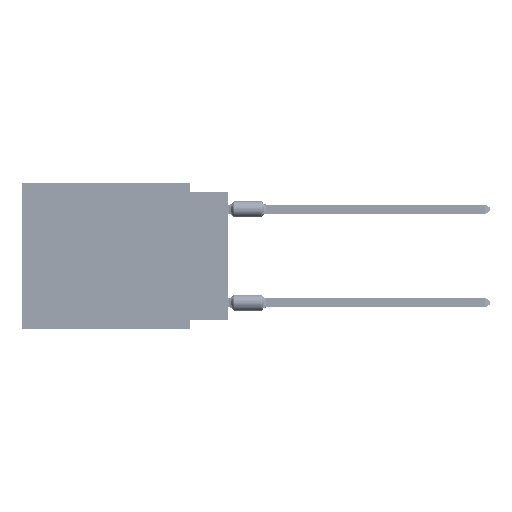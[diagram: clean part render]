
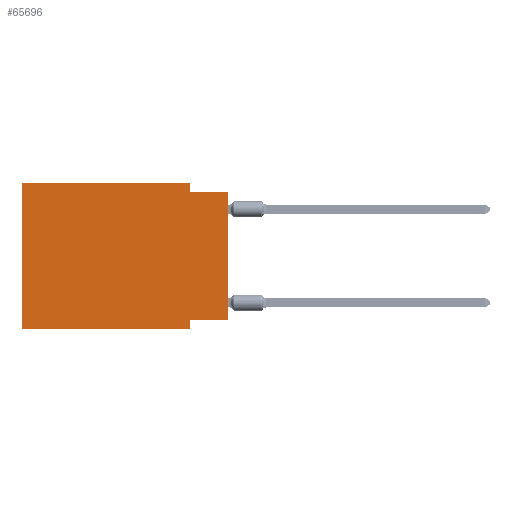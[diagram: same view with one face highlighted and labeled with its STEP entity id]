
A CAD part, left-side view. The second image highlights one B-rep face of the part: STEP entity #65696.
In plain terms, the highlighted planar face has unit normal (-1, 0, 0).
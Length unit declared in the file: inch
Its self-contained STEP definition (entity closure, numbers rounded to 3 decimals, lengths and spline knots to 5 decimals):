
#1277 = VECTOR ( 'NONE', #46324, 39.37008 ) ;
#2667 = EDGE_CURVE ( 'NONE', #44023, #79629, #66763, .T. ) ;
#2785 = VERTEX_POINT ( 'NONE', #69150 ) ;
#5005 = CARTESIAN_POINT ( 'NONE',  ( 0., 0.1, -0.39 ) ) ;
#6451 = CARTESIAN_POINT ( 'NONE',  ( 0., 0., -0.025 ) ) ;
#6894 = DIRECTION ( 'NONE',  ( 0., 0., -1. ) ) ;
#7888 = FACE_OUTER_BOUND ( 'NONE', #57667, .T. ) ;
#8982 = VECTOR ( 'NONE', #80253, 39.37008 ) ;
#9087 = CARTESIAN_POINT ( 'NONE',  ( 0., 0.55, -0.39 ) ) ;
#9197 = VERTEX_POINT ( 'NONE', #6451 ) ;
#11913 = CARTESIAN_POINT ( 'NONE',  ( 0., 0.1, -0.39 ) ) ;
#16998 = ORIENTED_EDGE ( 'NONE', *, *, #53743, .T. ) ;
#19771 = EDGE_CURVE ( 'NONE', #75054, #43557, #27640, .T. ) ;
#20317 = DIRECTION ( 'NONE',  ( 0., -1., 0. ) ) ;
#20482 = CARTESIAN_POINT ( 'NONE',  ( 0., 0.55, 0. ) ) ;
#20891 = ORIENTED_EDGE ( 'NONE', *, *, #31232, .T. ) ;
#21186 = CARTESIAN_POINT ( 'NONE',  ( 0., 0.55, -0.39 ) ) ;
#21458 = VERTEX_POINT ( 'NONE', #79711 ) ;
#21685 = VERTEX_POINT ( 'NONE', #21186 ) ;
#22049 = CARTESIAN_POINT ( 'NONE',  ( 0., 0.55, 0. ) ) ;
#22130 = CARTESIAN_POINT ( 'NONE',  ( 0., 0.1, -0.365 ) ) ;
#23485 = ORIENTED_EDGE ( 'NONE', *, *, #50300, .F. ) ;
#24976 = DIRECTION ( 'NONE',  ( 0., 0., -1. ) ) ;
#25943 = ORIENTED_EDGE ( 'NONE', *, *, #36119, .F. ) ;
#27640 = LINE ( 'NONE', #52410, #1277 ) ;
#31041 = LINE ( 'NONE', #42805, #70798 ) ;
#31232 = EDGE_CURVE ( 'NONE', #21458, #9197, #31041, .T. ) ;
#31469 = DIRECTION ( 'NONE',  ( 1., 0., 0. ) ) ;
#32112 = LINE ( 'NONE', #75944, #61336 ) ;
#32636 = VECTOR ( 'NONE', #52434, 39.37008 ) ;
#35011 = VECTOR ( 'NONE', #35903, 39.37008 ) ;
#35903 = DIRECTION ( 'NONE',  ( 0., 0., -1. ) ) ;
#36119 = EDGE_CURVE ( 'NONE', #21685, #75054, #77206, .T. ) ;
#37667 = EDGE_CURVE ( 'NONE', #2785, #9197, #32112, .T. ) ;
#38570 = LINE ( 'NONE', #68635, #79699 ) ;
#41069 = ORIENTED_EDGE ( 'NONE', *, *, #2667, .F. ) ;
#41079 = ORIENTED_EDGE ( 'NONE', *, *, #19771, .F. ) ;
#42036 = ORIENTED_EDGE ( 'NONE', *, *, #73039, .F. ) ;
#42805 = CARTESIAN_POINT ( 'NONE',  ( 0., 0., 0. ) ) ;
#43557 = VERTEX_POINT ( 'NONE', #51895 ) ;
#44023 = VERTEX_POINT ( 'NONE', #22130 ) ;
#45892 = LINE ( 'NONE', #61178, #8982 ) ;
#46324 = DIRECTION ( 'NONE',  ( 0., -1., 0. ) ) ;
#50300 = EDGE_CURVE ( 'NONE', #43557, #2785, #38570, .T. ) ;
#50542 = PLANE ( 'NONE',  #79718 ) ;
#51895 = CARTESIAN_POINT ( 'NONE',  ( 0., 0.1, 0. ) ) ;
#52410 = CARTESIAN_POINT ( 'NONE',  ( 0., 0.55, 0. ) ) ;
#52434 = DIRECTION ( 'NONE',  ( 0., 0., 1. ) ) ;
#53743 = EDGE_CURVE ( 'NONE', #21685, #79629, #58218, .T. ) ;
#55807 = DIRECTION ( 'NONE',  ( 0., 0., 1. ) ) ;
#57667 = EDGE_LOOP ( 'NONE', ( #20891, #70760, #23485, #41079, #25943, #16998, #41069, #42036 ) ) ;
#58218 = LINE ( 'NONE', #9087, #65632 ) ;
#61178 = CARTESIAN_POINT ( 'NONE',  ( 0., 0., -0.365 ) ) ;
#61336 = VECTOR ( 'NONE', #20317, 39.37008 ) ;
#65632 = VECTOR ( 'NONE', #70412, 39.37008 ) ;
#65696 = ADVANCED_FACE ( 'NONE', ( #7888 ), #50542, .F. ) ;
#66240 = CARTESIAN_POINT ( 'NONE',  ( 0., 0.55, 0. ) ) ;
#66763 = LINE ( 'NONE', #11913, #35011 ) ;
#68635 = CARTESIAN_POINT ( 'NONE',  ( 0., 0.1, 0. ) ) ;
#69150 = CARTESIAN_POINT ( 'NONE',  ( 0., 0.1, -0.025 ) ) ;
#70412 = DIRECTION ( 'NONE',  ( 0., -1., 0. ) ) ;
#70760 = ORIENTED_EDGE ( 'NONE', *, *, #37667, .F. ) ;
#70798 = VECTOR ( 'NONE', #55807, 39.37008 ) ;
#73039 = EDGE_CURVE ( 'NONE', #21458, #44023, #45892, .T. ) ;
#75054 = VERTEX_POINT ( 'NONE', #22049 ) ;
#75944 = CARTESIAN_POINT ( 'NONE',  ( 0., 0., -0.025 ) ) ;
#77206 = LINE ( 'NONE', #66240, #32636 ) ;
#79629 = VERTEX_POINT ( 'NONE', #5005 ) ;
#79699 = VECTOR ( 'NONE', #6894, 39.37008 ) ;
#79711 = CARTESIAN_POINT ( 'NONE',  ( 0., 0., -0.365 ) ) ;
#79718 = AXIS2_PLACEMENT_3D ( 'NONE', #20482, #31469, #24976 ) ;
#80253 = DIRECTION ( 'NONE',  ( 0., 1., 0. ) ) ;
